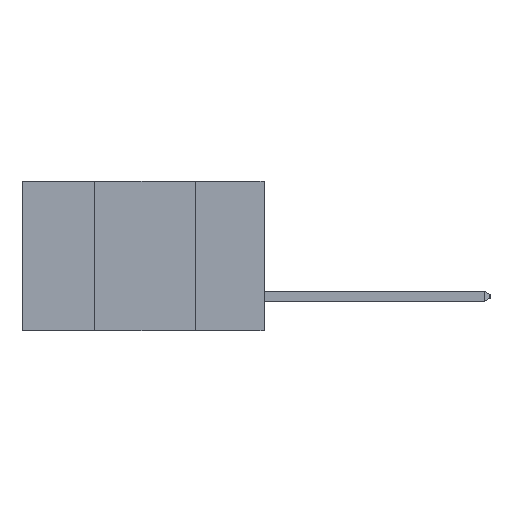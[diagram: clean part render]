
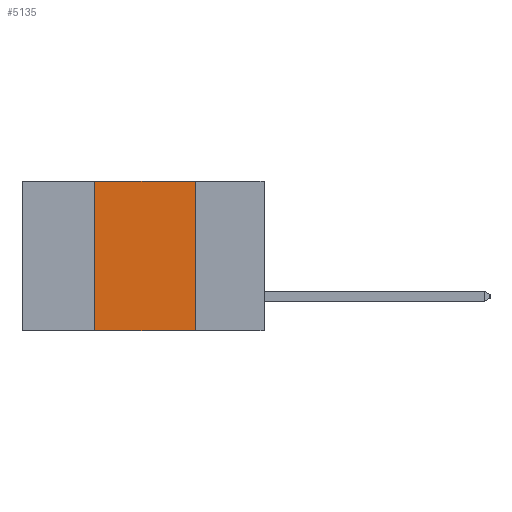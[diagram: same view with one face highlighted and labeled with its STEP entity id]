
A CAD part, left-side view. The second image highlights one B-rep face of the part: STEP entity #5135.
In plain terms, the highlighted planar face has unit normal (-1, 0, 0).
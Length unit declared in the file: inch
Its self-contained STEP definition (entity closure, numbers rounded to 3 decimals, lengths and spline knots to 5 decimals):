
#81 = EDGE_LOOP ( 'NONE', ( #9491, #6736, #8928, #11650 ) ) ;
#231 = DIRECTION ( 'NONE',  ( 0., -1., 0. ) ) ;
#291 = CARTESIAN_POINT ( 'NONE',  ( 0., 0.6, 0. ) ) ;
#674 = DIRECTION ( 'NONE',  ( 0., 0., -1. ) ) ;
#690 = DIRECTION ( 'NONE',  ( 1., 0., 0. ) ) ;
#706 = CARTESIAN_POINT ( 'NONE',  ( 0., 0.6, 0. ) ) ;
#794 = PLANE ( 'NONE',  #9274 ) ;
#1110 = VERTEX_POINT ( 'NONE', #7780 ) ;
#1304 = VECTOR ( 'NONE', #231, 39.37008 ) ;
#1315 = LINE ( 'NONE', #8666, #5788 ) ;
#1870 = EDGE_CURVE ( 'NONE', #5503, #2438, #9444, .T. ) ;
#2050 = VECTOR ( 'NONE', #2503, 39.37008 ) ;
#2154 = EDGE_CURVE ( 'NONE', #1110, #5503, #10666, .T. ) ;
#2206 = CARTESIAN_POINT ( 'NONE',  ( 0., 0.42, 0. ) ) ;
#2413 = LINE ( 'NONE', #2681, #2050 ) ;
#2438 = VERTEX_POINT ( 'NONE', #5108 ) ;
#2503 = DIRECTION ( 'NONE',  ( 0., -1., 0. ) ) ;
#2656 = EDGE_CURVE ( 'NONE', #1110, #7247, #2413, .T. ) ;
#2681 = CARTESIAN_POINT ( 'NONE',  ( 0., 0.6, -0.37 ) ) ;
#2914 = VECTOR ( 'NONE', #11585, 39.37008 ) ;
#3407 = EDGE_CURVE ( 'NONE', #2438, #7247, #1315, .T. ) ;
#4191 = CARTESIAN_POINT ( 'NONE',  ( 0., 0.17, -0.37 ) ) ;
#5108 = CARTESIAN_POINT ( 'NONE',  ( 0., 0.17, 0. ) ) ;
#5135 = ADVANCED_FACE ( 'NONE', ( #9242 ), #794, .F. ) ;
#5503 = VERTEX_POINT ( 'NONE', #2206 ) ;
#5788 = VECTOR ( 'NONE', #8444, 39.37008 ) ;
#6736 = ORIENTED_EDGE ( 'NONE', *, *, #1870, .F. ) ;
#7247 = VERTEX_POINT ( 'NONE', #4191 ) ;
#7780 = CARTESIAN_POINT ( 'NONE',  ( 0., 0.42, -0.37 ) ) ;
#8444 = DIRECTION ( 'NONE',  ( 0., 0., -1. ) ) ;
#8666 = CARTESIAN_POINT ( 'NONE',  ( 0., 0.17, -0.37 ) ) ;
#8928 = ORIENTED_EDGE ( 'NONE', *, *, #2154, .F. ) ;
#9242 = FACE_OUTER_BOUND ( 'NONE', #81, .T. ) ;
#9274 = AXIS2_PLACEMENT_3D ( 'NONE', #706, #690, #674 ) ;
#9444 = LINE ( 'NONE', #291, #1304 ) ;
#9491 = ORIENTED_EDGE ( 'NONE', *, *, #3407, .F. ) ;
#10666 = LINE ( 'NONE', #12053, #2914 ) ;
#11585 = DIRECTION ( 'NONE',  ( 0., 0., 1. ) ) ;
#11650 = ORIENTED_EDGE ( 'NONE', *, *, #2656, .T. ) ;
#12053 = CARTESIAN_POINT ( 'NONE',  ( 0., 0.42, -0.37 ) ) ;
